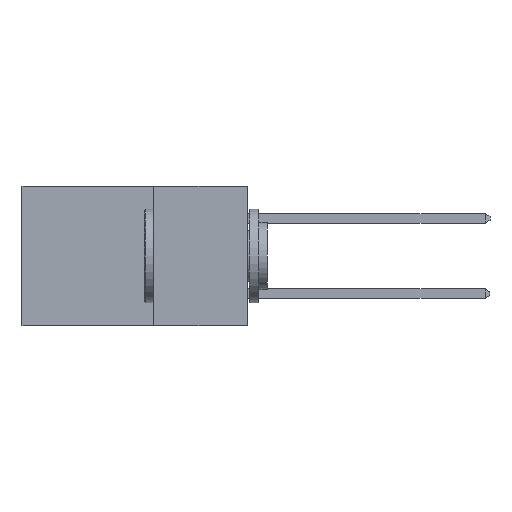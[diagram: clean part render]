
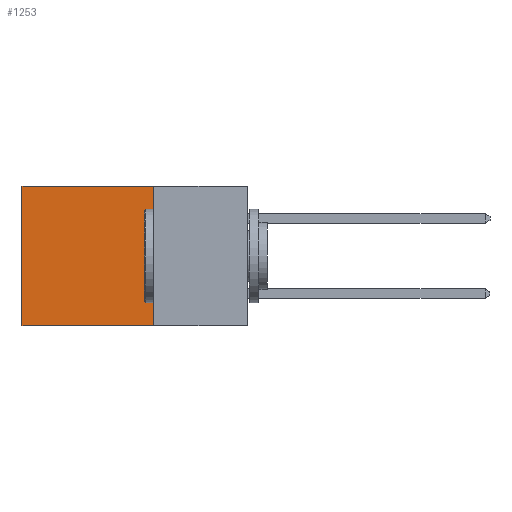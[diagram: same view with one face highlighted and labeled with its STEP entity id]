
A CAD part, left-side view. The second image highlights one B-rep face of the part: STEP entity #1253.
In plain terms, the highlighted planar face has unit normal (-1, 0, 0).
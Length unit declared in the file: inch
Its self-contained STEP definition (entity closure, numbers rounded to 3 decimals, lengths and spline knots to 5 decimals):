
#538 = FACE_OUTER_BOUND ( 'NONE', #7020, .T. ) ;
#600 = VECTOR ( 'NONE', #788, 39.37008 ) ;
#788 = DIRECTION ( 'NONE',  ( 0., 1., 0. ) ) ;
#956 = VECTOR ( 'NONE', #9794, 39.37008 ) ;
#1253 = ADVANCED_FACE ( 'NONE', ( #538 ), #7545, .F. ) ;
#1259 = VERTEX_POINT ( 'NONE', #7125 ) ;
#1954 = CARTESIAN_POINT ( 'NONE',  ( 0.298, 0.6, 0. ) ) ;
#2069 = CARTESIAN_POINT ( 'NONE',  ( 0.298, 0.25, 0. ) ) ;
#3775 = VECTOR ( 'NONE', #9282, 39.37008 ) ;
#3794 = VERTEX_POINT ( 'NONE', #14684 ) ;
#4218 = LINE ( 'NONE', #2069, #956 ) ;
#4231 = LINE ( 'NONE', #14591, #600 ) ;
#4273 = CARTESIAN_POINT ( 'NONE',  ( 0.298, 0.6, -0.37 ) ) ;
#4865 = ORIENTED_EDGE ( 'NONE', *, *, #15111, .T. ) ;
#4876 = LINE ( 'NONE', #9117, #8015 ) ;
#5214 = ORIENTED_EDGE ( 'NONE', *, *, #6100, .F. ) ;
#5710 = EDGE_CURVE ( 'NONE', #1259, #8346, #4231, .T. ) ;
#6100 = EDGE_CURVE ( 'NONE', #3794, #1259, #4218, .T. ) ;
#6879 = LINE ( 'NONE', #10405, #3775 ) ;
#7020 = EDGE_LOOP ( 'NONE', ( #10878, #11192, #5214, #4865 ) ) ;
#7088 = DIRECTION ( 'NONE',  ( 1., 0., 0. ) ) ;
#7125 = CARTESIAN_POINT ( 'NONE',  ( 0.298, 0.25, -0.37 ) ) ;
#7545 = PLANE ( 'NONE',  #11146 ) ;
#8015 = VECTOR ( 'NONE', #12616, 39.37008 ) ;
#8065 = DIRECTION ( 'NONE',  ( 0., 0., -1. ) ) ;
#8346 = VERTEX_POINT ( 'NONE', #4273 ) ;
#9117 = CARTESIAN_POINT ( 'NONE',  ( 0.298, 0.25, 0. ) ) ;
#9282 = DIRECTION ( 'NONE',  ( 0., 0., -1. ) ) ;
#9794 = DIRECTION ( 'NONE',  ( 0., 0., -1. ) ) ;
#10405 = CARTESIAN_POINT ( 'NONE',  ( 0.298, 0.6, 0. ) ) ;
#10878 = ORIENTED_EDGE ( 'NONE', *, *, #11736, .T. ) ;
#11146 = AXIS2_PLACEMENT_3D ( 'NONE', #13319, #7088, #8065 ) ;
#11192 = ORIENTED_EDGE ( 'NONE', *, *, #5710, .F. ) ;
#11689 = VERTEX_POINT ( 'NONE', #1954 ) ;
#11736 = EDGE_CURVE ( 'NONE', #11689, #8346, #6879, .T. ) ;
#12616 = DIRECTION ( 'NONE',  ( 0., 1., 0. ) ) ;
#13319 = CARTESIAN_POINT ( 'NONE',  ( 0.298, 0.25, 0. ) ) ;
#14591 = CARTESIAN_POINT ( 'NONE',  ( 0.298, 0.25, -0.37 ) ) ;
#14684 = CARTESIAN_POINT ( 'NONE',  ( 0.298, 0.25, 0. ) ) ;
#15111 = EDGE_CURVE ( 'NONE', #3794, #11689, #4876, .T. ) ;
